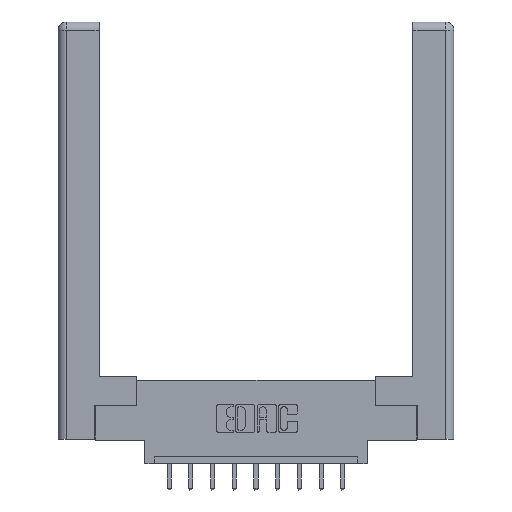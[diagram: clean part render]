
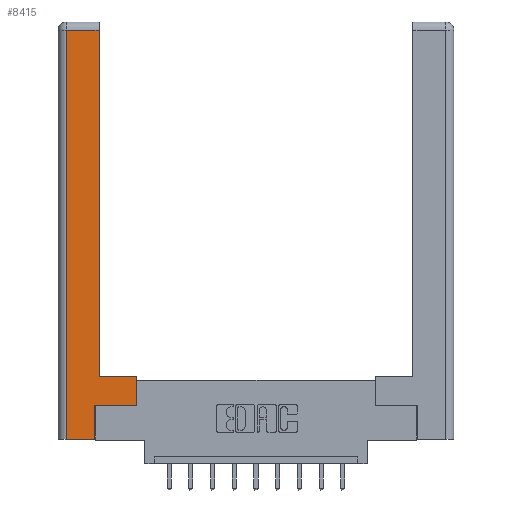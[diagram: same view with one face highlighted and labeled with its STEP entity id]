
A CAD part, top view. The second image highlights one B-rep face of the part: STEP entity #8415.
In plain terms, the highlighted planar face has unit normal (0, 0, 1).
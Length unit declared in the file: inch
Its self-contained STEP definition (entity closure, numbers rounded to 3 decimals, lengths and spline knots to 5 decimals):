
#50 = VERTEX_POINT ( 'NONE', #9121 ) ;
#104 = VERTEX_POINT ( 'NONE', #6841 ) ;
#171 = EDGE_CURVE ( 'NONE', #104, #12775, #7464, .T. ) ;
#463 = VECTOR ( 'NONE', #1659, 39.37008 ) ;
#579 = CARTESIAN_POINT ( 'NONE',  ( 0.0615, 2.94, 0. ) ) ;
#629 = DIRECTION ( 'NONE',  ( 0., 0., -1. ) ) ;
#757 = EDGE_CURVE ( 'NONE', #5387, #12873, #8637, .T. ) ;
#761 = LINE ( 'NONE', #12688, #8954 ) ;
#960 = LINE ( 'NONE', #7836, #3631 ) ;
#1104 = LINE ( 'NONE', #4910, #10169 ) ;
#1445 = CARTESIAN_POINT ( 'NONE',  ( 0.565, 0.45, 0. ) ) ;
#1659 = DIRECTION ( 'NONE',  ( -1., 0., 0. ) ) ;
#1889 = EDGE_CURVE ( 'NONE', #5354, #9753, #761, .T. ) ;
#1928 = LINE ( 'NONE', #13440, #11309 ) ;
#2263 = EDGE_CURVE ( 'NONE', #6946, #5387, #11631, .T. ) ;
#2305 = CARTESIAN_POINT ( 'NONE',  ( 0.265, 0., 0. ) ) ;
#2420 = EDGE_LOOP ( 'NONE', ( #11421, #4844, #3346, #3283, #6189, #8213, #4138, #3265 ) ) ;
#2456 = DIRECTION ( 'NONE',  ( 0., 1., 0. ) ) ;
#3265 = ORIENTED_EDGE ( 'NONE', *, *, #7999, .T. ) ;
#3283 = ORIENTED_EDGE ( 'NONE', *, *, #2263, .T. ) ;
#3346 = ORIENTED_EDGE ( 'NONE', *, *, #3966, .T. ) ;
#3631 = VECTOR ( 'NONE', #13269, 39.37008 ) ;
#3862 = CARTESIAN_POINT ( 'NONE',  ( 0.265, 0., 0. ) ) ;
#3966 = EDGE_CURVE ( 'NONE', #12775, #6946, #1104, .T. ) ;
#4138 = ORIENTED_EDGE ( 'NONE', *, *, #1889, .T. ) ;
#4256 = DIRECTION ( 'NONE',  ( 0., 1., 0. ) ) ;
#4441 = EDGE_CURVE ( 'NONE', #50, #104, #1928, .T. ) ;
#4689 = CARTESIAN_POINT ( 'NONE',  ( 0.295, 0.45, 0. ) ) ;
#4840 = PLANE ( 'NONE',  #13295 ) ;
#4844 = ORIENTED_EDGE ( 'NONE', *, *, #171, .T. ) ;
#4892 = LINE ( 'NONE', #4689, #7878 ) ;
#4910 = CARTESIAN_POINT ( 'NONE',  ( 0.0615, 0., 0. ) ) ;
#5354 = VERTEX_POINT ( 'NONE', #9890 ) ;
#5387 = VERTEX_POINT ( 'NONE', #2305 ) ;
#5905 = VECTOR ( 'NONE', #13407, 39.37008 ) ;
#5921 = DIRECTION ( 'NONE',  ( -1., 0., 0. ) ) ;
#6189 = ORIENTED_EDGE ( 'NONE', *, *, #757, .T. ) ;
#6841 = CARTESIAN_POINT ( 'NONE',  ( 0.295, 2.94, 0. ) ) ;
#6946 = VERTEX_POINT ( 'NONE', #13787 ) ;
#7013 = DIRECTION ( 'NONE',  ( 0., 1., 0. ) ) ;
#7464 = LINE ( 'NONE', #579, #463 ) ;
#7806 = DIRECTION ( 'NONE',  ( -1., 0., 0. ) ) ;
#7836 = CARTESIAN_POINT ( 'NONE',  ( 0.565, 0.245, 0. ) ) ;
#7878 = VECTOR ( 'NONE', #7806, 39.37008 ) ;
#7946 = CARTESIAN_POINT ( 'NONE',  ( 0., 0., 0. ) ) ;
#7999 = EDGE_CURVE ( 'NONE', #9753, #50, #4892, .T. ) ;
#8213 = ORIENTED_EDGE ( 'NONE', *, *, #10253, .T. ) ;
#8415 = ADVANCED_FACE ( 'NONE', ( #11741 ), #4840, .F. ) ;
#8637 = LINE ( 'NONE', #8762, #9841 ) ;
#8762 = CARTESIAN_POINT ( 'NONE',  ( 0.265, 0.245, 0. ) ) ;
#8954 = VECTOR ( 'NONE', #4256, 39.37008 ) ;
#9121 = CARTESIAN_POINT ( 'NONE',  ( 0.295, 0.45, 0. ) ) ;
#9604 = CARTESIAN_POINT ( 'NONE',  ( 0.0615, 2.94, 0. ) ) ;
#9753 = VERTEX_POINT ( 'NONE', #1445 ) ;
#9841 = VECTOR ( 'NONE', #2456, 39.37008 ) ;
#9890 = CARTESIAN_POINT ( 'NONE',  ( 0.565, 0.245, 0. ) ) ;
#10169 = VECTOR ( 'NONE', #10671, 39.37008 ) ;
#10253 = EDGE_CURVE ( 'NONE', #12873, #5354, #960, .T. ) ;
#10671 = DIRECTION ( 'NONE',  ( 0., -1., 0. ) ) ;
#11309 = VECTOR ( 'NONE', #7013, 39.37008 ) ;
#11421 = ORIENTED_EDGE ( 'NONE', *, *, #4441, .T. ) ;
#11631 = LINE ( 'NONE', #3862, #5905 ) ;
#11741 = FACE_OUTER_BOUND ( 'NONE', #2420, .T. ) ;
#12688 = CARTESIAN_POINT ( 'NONE',  ( 0.565, 0.45, 0. ) ) ;
#12775 = VERTEX_POINT ( 'NONE', #9604 ) ;
#12873 = VERTEX_POINT ( 'NONE', #13026 ) ;
#13026 = CARTESIAN_POINT ( 'NONE',  ( 0.265, 0.245, 0. ) ) ;
#13269 = DIRECTION ( 'NONE',  ( 1., 0., 0. ) ) ;
#13295 = AXIS2_PLACEMENT_3D ( 'NONE', #7946, #629, #5921 ) ;
#13407 = DIRECTION ( 'NONE',  ( 1., 0., 0. ) ) ;
#13440 = CARTESIAN_POINT ( 'NONE',  ( 0.295, 3., 0. ) ) ;
#13787 = CARTESIAN_POINT ( 'NONE',  ( 0.0615, 0., 0. ) ) ;
